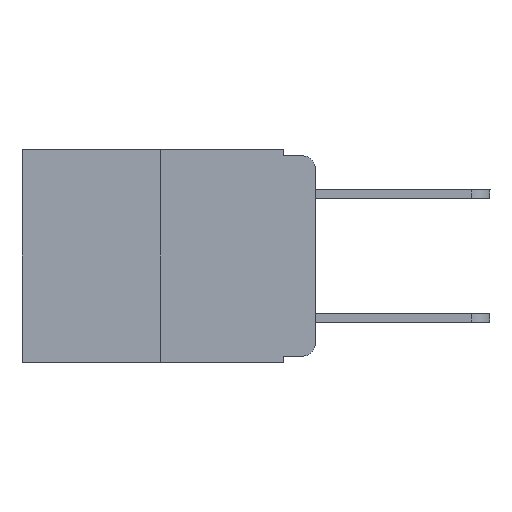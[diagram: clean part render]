
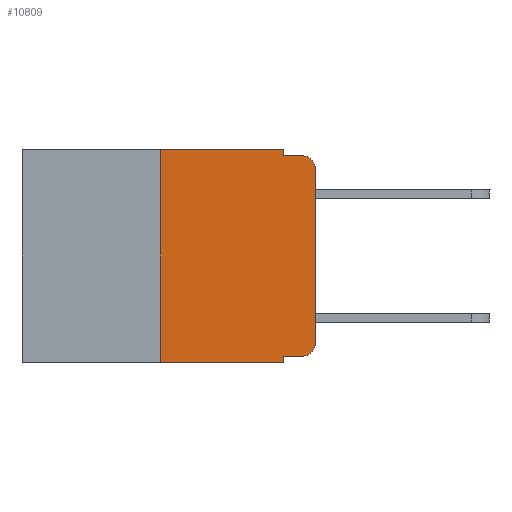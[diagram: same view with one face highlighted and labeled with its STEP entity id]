
A CAD part, left-side view. The second image highlights one B-rep face of the part: STEP entity #10809.
In plain terms, the highlighted planar face has unit normal (-1, 0, 0).
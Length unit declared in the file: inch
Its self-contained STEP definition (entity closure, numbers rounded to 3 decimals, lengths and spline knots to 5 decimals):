
#393 = VECTOR ( 'NONE', #17025, 39.37008 ) ;
#793 = DIRECTION ( 'NONE',  ( 0., 0., -1. ) ) ;
#1128 = FACE_OUTER_BOUND ( 'NONE', #10427, .T. ) ;
#1760 = DIRECTION ( 'NONE',  ( 0., -1., 0. ) ) ;
#1997 = VECTOR ( 'NONE', #13189, 39.37008 ) ;
#2400 = CIRCLE ( 'NONE', #11805, 0.02 ) ;
#2643 = DIRECTION ( 'NONE',  ( 0., 0., 1. ) ) ;
#2657 = CARTESIAN_POINT ( 'NONE',  ( 0., 0.02, -0.313 ) ) ;
#2950 = EDGE_CURVE ( 'NONE', #18196, #10447, #14714, .T. ) ;
#3435 = CARTESIAN_POINT ( 'NONE',  ( 0., 0.02, -0.01 ) ) ;
#3455 = CARTESIAN_POINT ( 'NONE',  ( 0., 0.051, 0. ) ) ;
#3474 = CARTESIAN_POINT ( 'NONE',  ( 0., 0.051, -0.343 ) ) ;
#3794 = CARTESIAN_POINT ( 'NONE',  ( 0., 0.051, -0.333 ) ) ;
#4052 = PLANE ( 'NONE',  #6685 ) ;
#4696 = CARTESIAN_POINT ( 'NONE',  ( 0., 0.051, 0. ) ) ;
#4724 = ORIENTED_EDGE ( 'NONE', *, *, #12635, .F. ) ;
#4808 = DIRECTION ( 'NONE',  ( 0., 0., -1. ) ) ;
#5426 = VERTEX_POINT ( 'NONE', #15432 ) ;
#5647 = CARTESIAN_POINT ( 'NONE',  ( 0., 0.473, 0. ) ) ;
#6457 = VECTOR ( 'NONE', #2643, 39.37008 ) ;
#6489 = ORIENTED_EDGE ( 'NONE', *, *, #9072, .F. ) ;
#6685 = AXIS2_PLACEMENT_3D ( 'NONE', #5647, #7022, #13001 ) ;
#6700 = ORIENTED_EDGE ( 'NONE', *, *, #11420, .T. ) ;
#7022 = DIRECTION ( 'NONE',  ( 1., 0., 0. ) ) ;
#7110 = CARTESIAN_POINT ( 'NONE',  ( 0., 0.473, -0.343 ) ) ;
#7496 = EDGE_CURVE ( 'NONE', #9030, #12149, #11203, .T. ) ;
#7860 = CARTESIAN_POINT ( 'NONE',  ( 0., 0.051, 0. ) ) ;
#7992 = VECTOR ( 'NONE', #11033, 39.37008 ) ;
#8519 = VECTOR ( 'NONE', #11492, 39.37008 ) ;
#8824 = DIRECTION ( 'NONE',  ( -1., 0., 0. ) ) ;
#9030 = VERTEX_POINT ( 'NONE', #13722 ) ;
#9072 = EDGE_CURVE ( 'NONE', #13562, #13027, #9603, .T. ) ;
#9179 = EDGE_CURVE ( 'NONE', #14580, #9030, #11357, .T. ) ;
#9209 = CARTESIAN_POINT ( 'NONE',  ( 0., 0., -0.313 ) ) ;
#9405 = CARTESIAN_POINT ( 'NONE',  ( 0., 0.051, -0.333 ) ) ;
#9461 = ORIENTED_EDGE ( 'NONE', *, *, #9179, .F. ) ;
#9603 = LINE ( 'NONE', #15281, #393 ) ;
#10427 = EDGE_LOOP ( 'NONE', ( #18394, #12788, #6489, #16355, #16205, #9461, #6700, #4724, #14173, #13808 ) ) ;
#10447 = VERTEX_POINT ( 'NONE', #9209 ) ;
#10451 = VECTOR ( 'NONE', #17128, 39.37008 ) ;
#10778 = LINE ( 'NONE', #9405, #13383 ) ;
#10809 = ADVANCED_FACE ( 'NONE', ( #1128 ), #4052, .F. ) ;
#11033 = DIRECTION ( 'NONE',  ( 0., 0., -1. ) ) ;
#11203 = LINE ( 'NONE', #11383, #8519 ) ;
#11241 = LINE ( 'NONE', #3455, #7992 ) ;
#11357 = LINE ( 'NONE', #18893, #10451 ) ;
#11383 = CARTESIAN_POINT ( 'NONE',  ( 0., 0.473, 0. ) ) ;
#11420 = EDGE_CURVE ( 'NONE', #14580, #16212, #14663, .T. ) ;
#11492 = DIRECTION ( 'NONE',  ( 0., -1., 0. ) ) ;
#11805 = AXIS2_PLACEMENT_3D ( 'NONE', #17716, #8824, #14893 ) ;
#12149 = VERTEX_POINT ( 'NONE', #4696 ) ;
#12170 = CARTESIAN_POINT ( 'NONE',  ( 0., 0.02, -0.333 ) ) ;
#12635 = EDGE_CURVE ( 'NONE', #17190, #16212, #11241, .T. ) ;
#12788 = ORIENTED_EDGE ( 'NONE', *, *, #13841, .T. ) ;
#12840 = AXIS2_PLACEMENT_3D ( 'NONE', #2657, #16079, #793 ) ;
#13001 = DIRECTION ( 'NONE',  ( 0., 0., -1. ) ) ;
#13027 = VERTEX_POINT ( 'NONE', #3435 ) ;
#13189 = DIRECTION ( 'NONE',  ( 0., -1., 0. ) ) ;
#13383 = VECTOR ( 'NONE', #1760, 39.37008 ) ;
#13562 = VERTEX_POINT ( 'NONE', #15592 ) ;
#13629 = EDGE_CURVE ( 'NONE', #10447, #5426, #19012, .T. ) ;
#13722 = CARTESIAN_POINT ( 'NONE',  ( 0., 0.25, 0. ) ) ;
#13808 = ORIENTED_EDGE ( 'NONE', *, *, #2950, .T. ) ;
#13841 = EDGE_CURVE ( 'NONE', #5426, #13027, #2400, .T. ) ;
#14173 = ORIENTED_EDGE ( 'NONE', *, *, #15713, .T. ) ;
#14417 = CARTESIAN_POINT ( 'NONE',  ( 0., 0., 0. ) ) ;
#14580 = VERTEX_POINT ( 'NONE', #16096 ) ;
#14663 = LINE ( 'NONE', #7110, #1997 ) ;
#14714 = CIRCLE ( 'NONE', #12840, 0.02 ) ;
#14893 = DIRECTION ( 'NONE',  ( 0., 0., -1. ) ) ;
#15169 = EDGE_CURVE ( 'NONE', #12149, #13562, #16495, .T. ) ;
#15281 = CARTESIAN_POINT ( 'NONE',  ( 0., 0.051, -0.01 ) ) ;
#15432 = CARTESIAN_POINT ( 'NONE',  ( 0., 0., -0.03 ) ) ;
#15592 = CARTESIAN_POINT ( 'NONE',  ( 0., 0.051, -0.01 ) ) ;
#15713 = EDGE_CURVE ( 'NONE', #17190, #18196, #10778, .T. ) ;
#16079 = DIRECTION ( 'NONE',  ( -1., 0., 0. ) ) ;
#16096 = CARTESIAN_POINT ( 'NONE',  ( 0., 0.25, -0.343 ) ) ;
#16205 = ORIENTED_EDGE ( 'NONE', *, *, #7496, .F. ) ;
#16212 = VERTEX_POINT ( 'NONE', #3474 ) ;
#16355 = ORIENTED_EDGE ( 'NONE', *, *, #15169, .F. ) ;
#16495 = LINE ( 'NONE', #7860, #16526 ) ;
#16526 = VECTOR ( 'NONE', #4808, 39.37008 ) ;
#17025 = DIRECTION ( 'NONE',  ( 0., -1., 0. ) ) ;
#17128 = DIRECTION ( 'NONE',  ( 0., 0., 1. ) ) ;
#17190 = VERTEX_POINT ( 'NONE', #3794 ) ;
#17716 = CARTESIAN_POINT ( 'NONE',  ( 0., 0.02, -0.03 ) ) ;
#18196 = VERTEX_POINT ( 'NONE', #12170 ) ;
#18394 = ORIENTED_EDGE ( 'NONE', *, *, #13629, .T. ) ;
#18893 = CARTESIAN_POINT ( 'NONE',  ( 0., 0.25, 0. ) ) ;
#19012 = LINE ( 'NONE', #14417, #6457 ) ;
